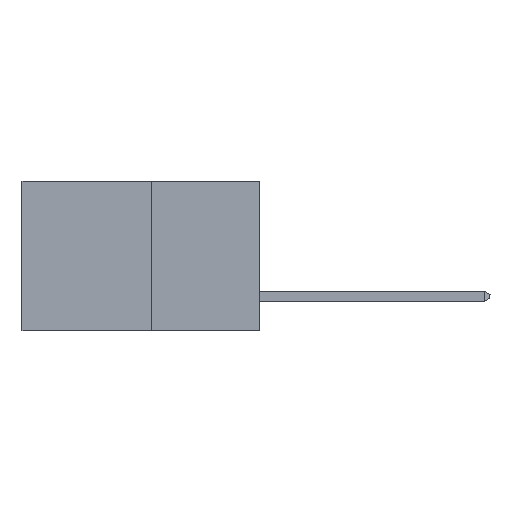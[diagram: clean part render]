
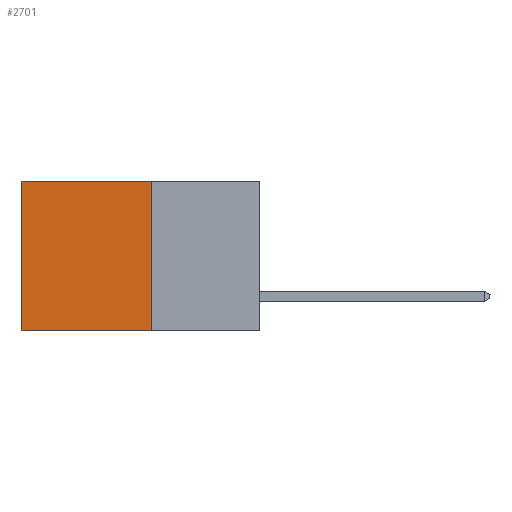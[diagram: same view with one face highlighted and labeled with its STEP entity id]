
A CAD part, left-side view. The second image highlights one B-rep face of the part: STEP entity #2701.
In plain terms, the highlighted planar face has unit normal (-1, 0, 0).
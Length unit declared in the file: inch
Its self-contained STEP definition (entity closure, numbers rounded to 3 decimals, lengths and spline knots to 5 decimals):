
#284 = VECTOR ( 'NONE', #8811, 39.37008 ) ;
#309 = CARTESIAN_POINT ( 'NONE',  ( 0.277, 0.27, -0.37 ) ) ;
#370 = CARTESIAN_POINT ( 'NONE',  ( 0.277, 0.59, -0.37 ) ) ;
#541 = LINE ( 'NONE', #1445, #284 ) ;
#837 = DIRECTION ( 'NONE',  ( 0., 0., -1. ) ) ;
#1280 = DIRECTION ( 'NONE',  ( 0., 1., 0. ) ) ;
#1445 = CARTESIAN_POINT ( 'NONE',  ( 0.277, 0.27, -0.37 ) ) ;
#1483 = ORIENTED_EDGE ( 'NONE', *, *, #2905, .T. ) ;
#2002 = ORIENTED_EDGE ( 'NONE', *, *, #9380, .T. ) ;
#2112 = VERTEX_POINT ( 'NONE', #3348 ) ;
#2234 = EDGE_LOOP ( 'NONE', ( #2002, #6449, #3505, #1483 ) ) ;
#2701 = ADVANCED_FACE ( 'NONE', ( #9328 ), #9376, .F. ) ;
#2905 = EDGE_CURVE ( 'NONE', #5567, #7102, #7555, .T. ) ;
#3186 = EDGE_CURVE ( 'NONE', #5567, #2112, #541, .T. ) ;
#3348 = CARTESIAN_POINT ( 'NONE',  ( 0.277, 0.27, -0.37 ) ) ;
#3505 = ORIENTED_EDGE ( 'NONE', *, *, #3186, .F. ) ;
#3911 = EDGE_CURVE ( 'NONE', #2112, #7006, #4223, .T. ) ;
#4071 = CARTESIAN_POINT ( 'NONE',  ( 0.277, 0.59, -0.37 ) ) ;
#4223 = LINE ( 'NONE', #9498, #9938 ) ;
#5233 = VECTOR ( 'NONE', #9721, 39.37008 ) ;
#5567 = VERTEX_POINT ( 'NONE', #9457 ) ;
#6449 = ORIENTED_EDGE ( 'NONE', *, *, #3911, .F. ) ;
#7006 = VERTEX_POINT ( 'NONE', #370 ) ;
#7102 = VERTEX_POINT ( 'NONE', #8815 ) ;
#7131 = DIRECTION ( 'NONE',  ( 0., 0., -1. ) ) ;
#7156 = VECTOR ( 'NONE', #837, 39.37008 ) ;
#7186 = DIRECTION ( 'NONE',  ( 1., 0., 0. ) ) ;
#7555 = LINE ( 'NONE', #7965, #5233 ) ;
#7965 = CARTESIAN_POINT ( 'NONE',  ( 0.277, 0.27, 0. ) ) ;
#8014 = AXIS2_PLACEMENT_3D ( 'NONE', #309, #7186, #7131 ) ;
#8811 = DIRECTION ( 'NONE',  ( 0., 0., -1. ) ) ;
#8815 = CARTESIAN_POINT ( 'NONE',  ( 0.277, 0.59, 0. ) ) ;
#9259 = LINE ( 'NONE', #4071, #7156 ) ;
#9328 = FACE_OUTER_BOUND ( 'NONE', #2234, .T. ) ;
#9376 = PLANE ( 'NONE',  #8014 ) ;
#9380 = EDGE_CURVE ( 'NONE', #7102, #7006, #9259, .T. ) ;
#9457 = CARTESIAN_POINT ( 'NONE',  ( 0.277, 0.27, 0. ) ) ;
#9498 = CARTESIAN_POINT ( 'NONE',  ( 0.277, 0.27, -0.37 ) ) ;
#9721 = DIRECTION ( 'NONE',  ( 0., 1., 0. ) ) ;
#9938 = VECTOR ( 'NONE', #1280, 39.37008 ) ;
